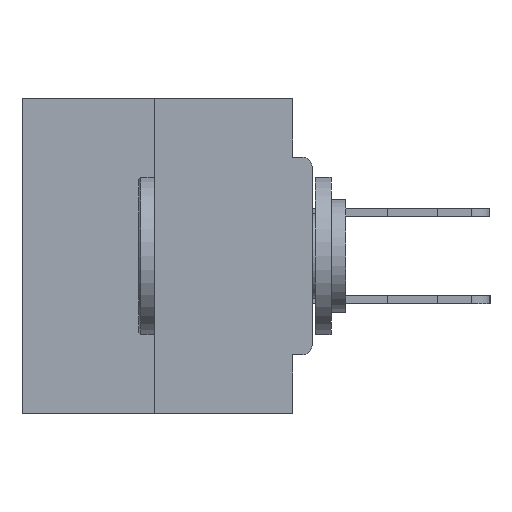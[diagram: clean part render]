
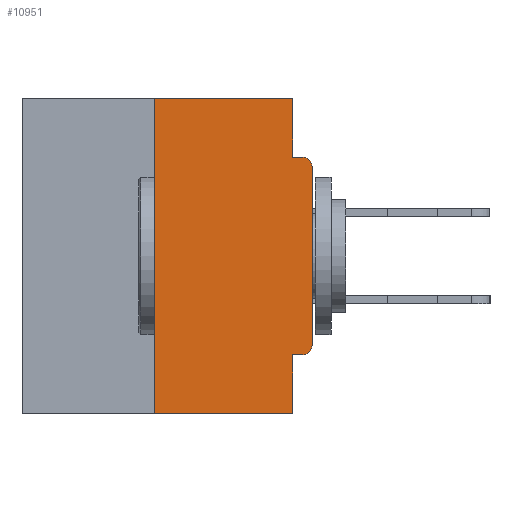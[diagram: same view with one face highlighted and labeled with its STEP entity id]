
A CAD part, left-side view. The second image highlights one B-rep face of the part: STEP entity #10951.
In plain terms, the highlighted planar face has unit normal (-1, 0, 0).
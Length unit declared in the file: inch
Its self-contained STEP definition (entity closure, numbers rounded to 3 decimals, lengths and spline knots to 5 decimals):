
#1164 = VERTEX_POINT ( 'NONE', #28581 ) ;
#1423 = CARTESIAN_POINT ( 'NONE',  ( 0., 0., 0. ) ) ;
#1467 = FACE_OUTER_BOUND ( 'NONE', #20098, .T. ) ;
#1871 = DIRECTION ( 'NONE',  ( 0., 0., -1. ) ) ;
#1962 = PLANE ( 'NONE',  #37026 ) ;
#2461 = DIRECTION ( 'NONE',  ( 0., 0., -1. ) ) ;
#3264 = EDGE_CURVE ( 'NONE', #11745, #14120, #38401, .T. ) ;
#3480 = VERTEX_POINT ( 'NONE', #10952 ) ;
#4842 = DIRECTION ( 'NONE',  ( 1., 0., 0. ) ) ;
#5236 = VECTOR ( 'NONE', #37641, 39.37008 ) ;
#6320 = CIRCLE ( 'NONE', #8964, 0.015 ) ;
#6772 = CARTESIAN_POINT ( 'NONE',  ( 0., 0.46, -0.5 ) ) ;
#6926 = LINE ( 'NONE', #25726, #18677 ) ;
#7177 = CARTESIAN_POINT ( 'NONE',  ( 0., 0.031, -0.4065 ) ) ;
#7609 = DIRECTION ( 'NONE',  ( 0., -1., 0. ) ) ;
#7983 = CARTESIAN_POINT ( 'NONE',  ( 0., 0.46, 0. ) ) ;
#8182 = DIRECTION ( 'NONE',  ( 0., 0., 1. ) ) ;
#8321 = EDGE_CURVE ( 'NONE', #3480, #35445, #24908, .T. ) ;
#8622 = CARTESIAN_POINT ( 'NONE',  ( 0., 0.031, 0. ) ) ;
#8964 = AXIS2_PLACEMENT_3D ( 'NONE', #16819, #14049, #1871 ) ;
#10937 = CARTESIAN_POINT ( 'NONE',  ( 0., 0.031, 0. ) ) ;
#10951 = ADVANCED_FACE ( 'NONE', ( #1467 ), #1962, .F. ) ;
#10952 = CARTESIAN_POINT ( 'NONE',  ( 0., 0.25, 0. ) ) ;
#11603 = VECTOR ( 'NONE', #27503, 39.37008 ) ;
#11745 = VERTEX_POINT ( 'NONE', #17766 ) ;
#12179 = EDGE_CURVE ( 'NONE', #35445, #37566, #34717, .T. ) ;
#13259 = CARTESIAN_POINT ( 'NONE',  ( 0., 0.46, 0. ) ) ;
#13693 = ORIENTED_EDGE ( 'NONE', *, *, #33120, .F. ) ;
#13893 = ORIENTED_EDGE ( 'NONE', *, *, #29043, .T. ) ;
#13977 = ORIENTED_EDGE ( 'NONE', *, *, #12179, .F. ) ;
#14049 = DIRECTION ( 'NONE',  ( -1., 0., 0. ) ) ;
#14120 = VERTEX_POINT ( 'NONE', #23789 ) ;
#16819 = CARTESIAN_POINT ( 'NONE',  ( 0., 0.015, -0.3915 ) ) ;
#16902 = AXIS2_PLACEMENT_3D ( 'NONE', #32558, #29276, #29148 ) ;
#16955 = VERTEX_POINT ( 'NONE', #28072 ) ;
#16970 = VECTOR ( 'NONE', #7609, 39.37008 ) ;
#17766 = CARTESIAN_POINT ( 'NONE',  ( 0., 0.25, -0.5 ) ) ;
#17776 = VECTOR ( 'NONE', #25836, 39.37008 ) ;
#18406 = VECTOR ( 'NONE', #27426, 39.37008 ) ;
#18524 = CARTESIAN_POINT ( 'NONE',  ( 0., 0.031, -0.5 ) ) ;
#18601 = EDGE_CURVE ( 'NONE', #11745, #3480, #30222, .T. ) ;
#18677 = VECTOR ( 'NONE', #34302, 39.37008 ) ;
#18978 = VECTOR ( 'NONE', #8182, 39.37008 ) ;
#20098 = EDGE_LOOP ( 'NONE', ( #26446, #29443, #20292, #35201, #13693, #13893, #33356, #28962, #26579, #13977 ) ) ;
#20226 = CARTESIAN_POINT ( 'NONE',  ( 0., 0.031, -0.0935 ) ) ;
#20292 = ORIENTED_EDGE ( 'NONE', *, *, #3264, .T. ) ;
#22127 = LINE ( 'NONE', #1423, #5236 ) ;
#22162 = LINE ( 'NONE', #18524, #18406 ) ;
#22235 = VERTEX_POINT ( 'NONE', #34354 ) ;
#22619 = EDGE_CURVE ( 'NONE', #37566, #22235, #6926, .T. ) ;
#23131 = CARTESIAN_POINT ( 'NONE',  ( 0., 0.25, 0. ) ) ;
#23789 = CARTESIAN_POINT ( 'NONE',  ( 0., 0.031, -0.5 ) ) ;
#24030 = CARTESIAN_POINT ( 'NONE',  ( 0., 0., -0.1085 ) ) ;
#24507 = EDGE_CURVE ( 'NONE', #31034, #14120, #22162, .T. ) ;
#24777 = EDGE_CURVE ( 'NONE', #1164, #32752, #22127, .T. ) ;
#24908 = LINE ( 'NONE', #13259, #16970 ) ;
#25726 = CARTESIAN_POINT ( 'NONE',  ( 0., 0., -0.0935 ) ) ;
#25836 = DIRECTION ( 'NONE',  ( 0., 1., 0. ) ) ;
#26202 = CIRCLE ( 'NONE', #16902, 0.015 ) ;
#26446 = ORIENTED_EDGE ( 'NONE', *, *, #8321, .F. ) ;
#26579 = ORIENTED_EDGE ( 'NONE', *, *, #22619, .F. ) ;
#26678 = VECTOR ( 'NONE', #2461, 39.37008 ) ;
#27426 = DIRECTION ( 'NONE',  ( 0., 0., -1. ) ) ;
#27503 = DIRECTION ( 'NONE',  ( 0., -1., 0. ) ) ;
#28072 = CARTESIAN_POINT ( 'NONE',  ( 0., 0.015, -0.4065 ) ) ;
#28581 = CARTESIAN_POINT ( 'NONE',  ( 0., 0., -0.3915 ) ) ;
#28717 = DIRECTION ( 'NONE',  ( 0., 0., -1. ) ) ;
#28962 = ORIENTED_EDGE ( 'NONE', *, *, #34212, .T. ) ;
#29043 = EDGE_CURVE ( 'NONE', #16955, #1164, #6320, .T. ) ;
#29148 = DIRECTION ( 'NONE',  ( 0., 0., -1. ) ) ;
#29276 = DIRECTION ( 'NONE',  ( -1., 0., 0. ) ) ;
#29443 = ORIENTED_EDGE ( 'NONE', *, *, #18601, .F. ) ;
#30222 = LINE ( 'NONE', #23131, #18978 ) ;
#30476 = LINE ( 'NONE', #31922, #17776 ) ;
#31034 = VERTEX_POINT ( 'NONE', #7177 ) ;
#31922 = CARTESIAN_POINT ( 'NONE',  ( 0., 0., -0.4065 ) ) ;
#32558 = CARTESIAN_POINT ( 'NONE',  ( 0., 0.015, -0.1085 ) ) ;
#32752 = VERTEX_POINT ( 'NONE', #24030 ) ;
#33120 = EDGE_CURVE ( 'NONE', #16955, #31034, #30476, .T. ) ;
#33356 = ORIENTED_EDGE ( 'NONE', *, *, #24777, .T. ) ;
#34212 = EDGE_CURVE ( 'NONE', #32752, #22235, #26202, .T. ) ;
#34302 = DIRECTION ( 'NONE',  ( 0., -1., 0. ) ) ;
#34354 = CARTESIAN_POINT ( 'NONE',  ( 0., 0.015, -0.0935 ) ) ;
#34717 = LINE ( 'NONE', #8622, #26678 ) ;
#35201 = ORIENTED_EDGE ( 'NONE', *, *, #24507, .F. ) ;
#35445 = VERTEX_POINT ( 'NONE', #10937 ) ;
#37026 = AXIS2_PLACEMENT_3D ( 'NONE', #7983, #4842, #28717 ) ;
#37566 = VERTEX_POINT ( 'NONE', #20226 ) ;
#37641 = DIRECTION ( 'NONE',  ( 0., 0., 1. ) ) ;
#38401 = LINE ( 'NONE', #6772, #11603 ) ;
